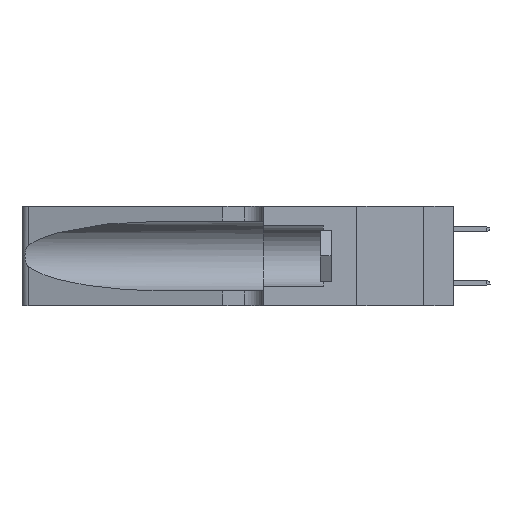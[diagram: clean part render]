
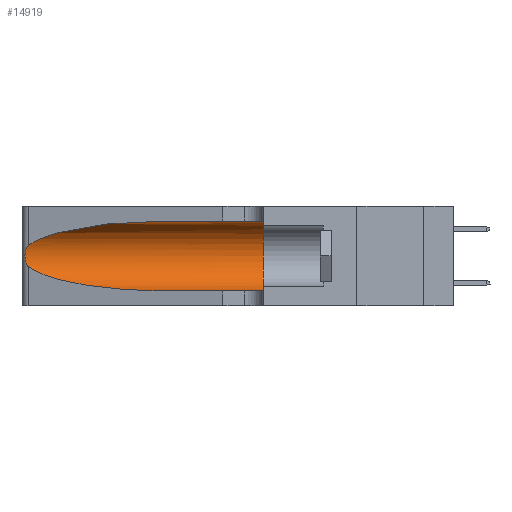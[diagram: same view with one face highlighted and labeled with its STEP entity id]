
A CAD part, left-side view. The second image highlights one B-rep face of the part: STEP entity #14919.
In plain terms, the highlighted cylindrical face has radius 3.308 mm (diameter 6.617 mm), a partial arc.
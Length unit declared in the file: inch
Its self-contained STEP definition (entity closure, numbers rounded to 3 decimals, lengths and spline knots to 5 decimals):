
#2 = DIRECTION ( 'NONE',  ( 0., -1., 0. ) ) ;
#248 = DIRECTION ( 'NONE',  ( 0., -1., 0. ) ) ;
#453 = CARTESIAN_POINT ( 'NONE',  ( 0.25787, 1.23484, 0.2124 ) ) ;
#509 = CARTESIAN_POINT ( 'NONE',  ( 0.1305, 0.72297, 0.31525 ) ) ;
#733 = CARTESIAN_POINT ( 'NONE',  ( 0.26075, 1.23896, 0.178 ) ) ;
#754 = CARTESIAN_POINT ( 'NONE',  ( 0.1305, 0.35, 0.31525 ) ) ;
#788 = EDGE_CURVE ( 'NONE', #3374, #16441, #14451, .T. ) ;
#1175 = VERTEX_POINT ( 'NONE', #754 ) ;
#1415 = EDGE_CURVE ( 'NONE', #9173, #17649, #6309, .T. ) ;
#1578 = CARTESIAN_POINT ( 'NONE',  ( 0.25487, 1.22718, 0.22369 ) ) ;
#1653 = LINE ( 'NONE', #10268, #17970 ) ;
#1938 = CARTESIAN_POINT ( 'NONE',  ( 0.25856, 1.23593, 0.16098 ) ) ;
#2706 = CARTESIAN_POINT ( 'NONE',  ( 0.1305, 1.61858, 0.185 ) ) ;
#2872 = CARTESIAN_POINT ( 'NONE',  ( 0.2373, 1.15595, 0.28018 ) ) ;
#3374 = VERTEX_POINT ( 'NONE', #14585 ) ;
#3436 = CARTESIAN_POINT ( 'NONE',  ( 0.25555, 1.22994, 0.2215 ) ) ;
#3549 = EDGE_CURVE ( 'NONE', #16441, #3706, #1653, .T. ) ;
#3706 = VERTEX_POINT ( 'NONE', #4914 ) ;
#3776 = EDGE_CURVE ( 'NONE', #1175, #3706, #9036, .T. ) ;
#4374 = ORIENTED_EDGE ( 'NONE', *, *, #3776, .F. ) ;
#4852 = AXIS2_PLACEMENT_3D ( 'NONE', #12855, #5743, #11468 ) ;
#4914 = CARTESIAN_POINT ( 'NONE',  ( 0.1305, 0.35, 0.05475 ) ) ;
#4922 = CARTESIAN_POINT ( 'NONE',  ( 0.26017, 1.23833, 0.17102 ) ) ;
#5151 = EDGE_CURVE ( 'NONE', #9173, #1175, #5856, .T. ) ;
#5338 = ORIENTED_EDGE ( 'NONE', *, *, #3549, .T. ) ;
#5504 = CARTESIAN_POINT ( 'NONE',  ( 0.1305, 0.72297, 0.31525 ) ) ;
#5743 = DIRECTION ( 'NONE',  ( 0., 1., 0. ) ) ;
#5856 = LINE ( 'NONE', #12979, #18236 ) ;
#5948 = DIRECTION ( 'NONE',  ( 0., -1., 0. ) ) ;
#6087 = CARTESIAN_POINT ( 'NONE',  ( 0.1305, 0.72297, 0.05475 ) ) ;
#6309 =( BOUNDED_CURVE ( )  B_SPLINE_CURVE ( 3, ( #5504, #6909, #2872, #1578 ),
 .UNSPECIFIED., .F., .T. ) 
 B_SPLINE_CURVE_WITH_KNOTS ( ( 4, 4 ),
 ( 1.5708, 2.84003 ),
 .UNSPECIFIED. ) 
 CURVE ( )  GEOMETRIC_REPRESENTATION_ITEM ( )  RATIONAL_B_SPLINE_CURVE ( ( 1., 0.87, 0.87, 1. ) ) 
 REPRESENTATION_ITEM ( '' )  );
#6909 = CARTESIAN_POINT ( 'NONE',  ( 0.18966, 0.96281, 0.31525 ) ) ;
#7096 = CYLINDRICAL_SURFACE ( 'NONE', #18159, 0.13025 ) ;
#7245 = B_SPLINE_CURVE_WITH_KNOTS ( 'NONE', 3,
 ( #14765, #3436, #8945, #453, #17616, #9327, #13249, #733, #4922, #1938, #9125, #10731, #13340, #17527 ),
 .UNSPECIFIED., .F., .F.,
 ( 4, 2, 2, 2, 2, 2, 4 ),
 ( 0., 0.00027, 0.00053, 0.00107, 0.0016, 0.00187, 0.00214 ),
 .UNSPECIFIED. ) ;
#7415 = CARTESIAN_POINT ( 'NONE',  ( 0.25487, 1.22718, 0.22369 ) ) ;
#7803 = EDGE_CURVE ( 'NONE', #17649, #3374, #7245, .T. ) ;
#8945 = CARTESIAN_POINT ( 'NONE',  ( 0.25639, 1.23184, 0.21858 ) ) ;
#9036 = CIRCLE ( 'NONE', #4852, 0.13025 ) ;
#9059 = CARTESIAN_POINT ( 'NONE',  ( 0.18966, 0.96281, 0.05475 ) ) ;
#9125 = CARTESIAN_POINT ( 'NONE',  ( 0.25789, 1.23486, 0.15765 ) ) ;
#9173 = VERTEX_POINT ( 'NONE', #509 ) ;
#9327 = CARTESIAN_POINT ( 'NONE',  ( 0.26018, 1.23835, 0.19895 ) ) ;
#9640 = ORIENTED_EDGE ( 'NONE', *, *, #788, .T. ) ;
#10268 = CARTESIAN_POINT ( 'NONE',  ( 0.1305, 1.61858, 0.05475 ) ) ;
#10472 = CARTESIAN_POINT ( 'NONE',  ( 0.25487, 1.22718, 0.14631 ) ) ;
#10690 = EDGE_LOOP ( 'NONE', ( #15744, #14611, #9640, #5338, #4374, #17963 ) ) ;
#10731 = CARTESIAN_POINT ( 'NONE',  ( 0.25639, 1.23186, 0.15144 ) ) ;
#11468 = DIRECTION ( 'NONE',  ( 0., 0., 1. ) ) ;
#12855 = CARTESIAN_POINT ( 'NONE',  ( 0.1305, 0.35, 0.185 ) ) ;
#12894 = DIRECTION ( 'NONE',  ( 0., 0., -1. ) ) ;
#12979 = CARTESIAN_POINT ( 'NONE',  ( 0.1305, 1.61858, 0.31525 ) ) ;
#12987 = FACE_OUTER_BOUND ( 'NONE', #10690, .T. ) ;
#13249 = CARTESIAN_POINT ( 'NONE',  ( 0.26075, 1.23896, 0.19203 ) ) ;
#13340 = CARTESIAN_POINT ( 'NONE',  ( 0.25555, 1.22993, 0.14849 ) ) ;
#14451 =( BOUNDED_CURVE ( )  B_SPLINE_CURVE ( 3, ( #10472, #16167, #9059, #14781 ),
 .UNSPECIFIED., .F., .T. ) 
 B_SPLINE_CURVE_WITH_KNOTS ( ( 4, 4 ),
 ( 3.44316, 4.71239 ),
 .UNSPECIFIED. ) 
 CURVE ( )  GEOMETRIC_REPRESENTATION_ITEM ( )  RATIONAL_B_SPLINE_CURVE ( ( 1., 0.87, 0.87, 1. ) ) 
 REPRESENTATION_ITEM ( '' )  );
#14585 = CARTESIAN_POINT ( 'NONE',  ( 0.25487, 1.22718, 0.14631 ) ) ;
#14611 = ORIENTED_EDGE ( 'NONE', *, *, #7803, .T. ) ;
#14765 = CARTESIAN_POINT ( 'NONE',  ( 0.25487, 1.22718, 0.22369 ) ) ;
#14781 = CARTESIAN_POINT ( 'NONE',  ( 0.1305, 0.72297, 0.05475 ) ) ;
#14919 = ADVANCED_FACE ( 'NONE', ( #12987 ), #7096, .F. ) ;
#15744 = ORIENTED_EDGE ( 'NONE', *, *, #1415, .T. ) ;
#16167 = CARTESIAN_POINT ( 'NONE',  ( 0.2373, 1.15595, 0.08982 ) ) ;
#16441 = VERTEX_POINT ( 'NONE', #6087 ) ;
#17527 = CARTESIAN_POINT ( 'NONE',  ( 0.25487, 1.22718, 0.14631 ) ) ;
#17616 = CARTESIAN_POINT ( 'NONE',  ( 0.25854, 1.2359, 0.20912 ) ) ;
#17649 = VERTEX_POINT ( 'NONE', #7415 ) ;
#17963 = ORIENTED_EDGE ( 'NONE', *, *, #5151, .F. ) ;
#17970 = VECTOR ( 'NONE', #248, 39.37008 ) ;
#18159 = AXIS2_PLACEMENT_3D ( 'NONE', #2706, #2, #12894 ) ;
#18236 = VECTOR ( 'NONE', #5948, 39.37008 ) ;
